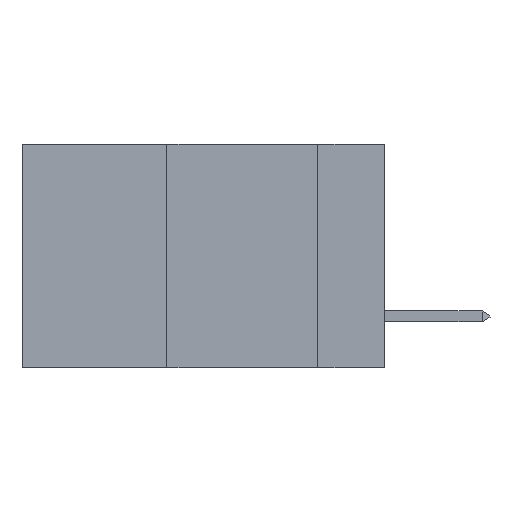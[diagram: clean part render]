
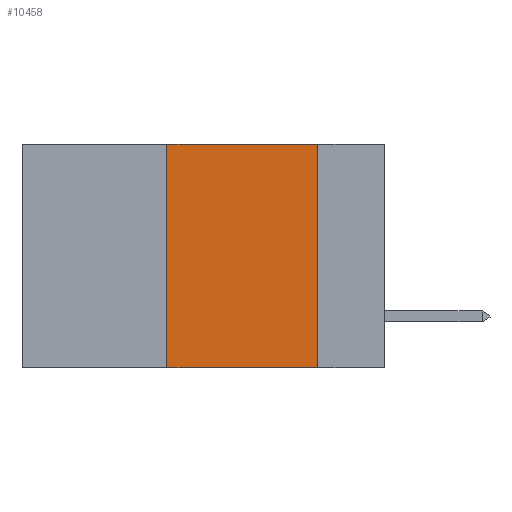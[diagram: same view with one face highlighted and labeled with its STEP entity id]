
A CAD part, left-side view. The second image highlights one B-rep face of the part: STEP entity #10458.
In plain terms, the highlighted planar face has unit normal (-1, 0, 0).
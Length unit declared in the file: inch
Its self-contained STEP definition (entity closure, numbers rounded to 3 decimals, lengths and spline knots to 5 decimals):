
#444 = LINE ( 'NONE', #11660, #16836 ) ;
#1110 = VERTEX_POINT ( 'NONE', #16970 ) ;
#2812 = CARTESIAN_POINT ( 'NONE',  ( 0., 0.36, 0. ) ) ;
#3941 = DIRECTION ( 'NONE',  ( 0., 0., 1. ) ) ;
#5529 = CARTESIAN_POINT ( 'NONE',  ( 0., 0.11, 0. ) ) ;
#6319 = LINE ( 'NONE', #15012, #16655 ) ;
#6585 = LINE ( 'NONE', #14074, #11608 ) ;
#7164 = AXIS2_PLACEMENT_3D ( 'NONE', #7330, #15847, #9046 ) ;
#7330 = CARTESIAN_POINT ( 'NONE',  ( 0., 0.6, 0. ) ) ;
#7693 = EDGE_CURVE ( 'NONE', #21680, #1110, #6319, .T. ) ;
#8125 = DIRECTION ( 'NONE',  ( 0., -1., 0. ) ) ;
#8415 = DIRECTION ( 'NONE',  ( 0., -1., 0. ) ) ;
#9046 = DIRECTION ( 'NONE',  ( 0., 0., -1. ) ) ;
#10458 = ADVANCED_FACE ( 'NONE', ( #13499 ), #17498, .F. ) ;
#10988 = CARTESIAN_POINT ( 'NONE',  ( 0., 0.11, 0. ) ) ;
#11200 = ORIENTED_EDGE ( 'NONE', *, *, #16807, .F. ) ;
#11608 = VECTOR ( 'NONE', #3941, 39.37008 ) ;
#11660 = CARTESIAN_POINT ( 'NONE',  ( 0., 0.6, 0. ) ) ;
#13499 = FACE_OUTER_BOUND ( 'NONE', #21475, .T. ) ;
#13796 = VERTEX_POINT ( 'NONE', #2812 ) ;
#14074 = CARTESIAN_POINT ( 'NONE',  ( 0., 0.36, 0. ) ) ;
#14112 = DIRECTION ( 'NONE',  ( 0., 0., -1. ) ) ;
#14910 = EDGE_CURVE ( 'NONE', #21680, #13796, #6585, .T. ) ;
#15012 = CARTESIAN_POINT ( 'NONE',  ( 0., 0.6, -0.37 ) ) ;
#15323 = LINE ( 'NONE', #10988, #17723 ) ;
#15793 = ORIENTED_EDGE ( 'NONE', *, *, #7693, .T. ) ;
#15847 = DIRECTION ( 'NONE',  ( 1., 0., 0. ) ) ;
#16655 = VECTOR ( 'NONE', #8125, 39.37008 ) ;
#16807 = EDGE_CURVE ( 'NONE', #13796, #20131, #444, .T. ) ;
#16836 = VECTOR ( 'NONE', #8415, 39.37008 ) ;
#16970 = CARTESIAN_POINT ( 'NONE',  ( 0., 0.11, -0.37 ) ) ;
#17498 = PLANE ( 'NONE',  #7164 ) ;
#17723 = VECTOR ( 'NONE', #14112, 39.37008 ) ;
#20131 = VERTEX_POINT ( 'NONE', #5529 ) ;
#20252 = EDGE_CURVE ( 'NONE', #20131, #1110, #15323, .T. ) ;
#21006 = ORIENTED_EDGE ( 'NONE', *, *, #14910, .F. ) ;
#21185 = ORIENTED_EDGE ( 'NONE', *, *, #20252, .F. ) ;
#21475 = EDGE_LOOP ( 'NONE', ( #21185, #11200, #21006, #15793 ) ) ;
#21661 = CARTESIAN_POINT ( 'NONE',  ( 0., 0.36, -0.37 ) ) ;
#21680 = VERTEX_POINT ( 'NONE', #21661 ) ;
